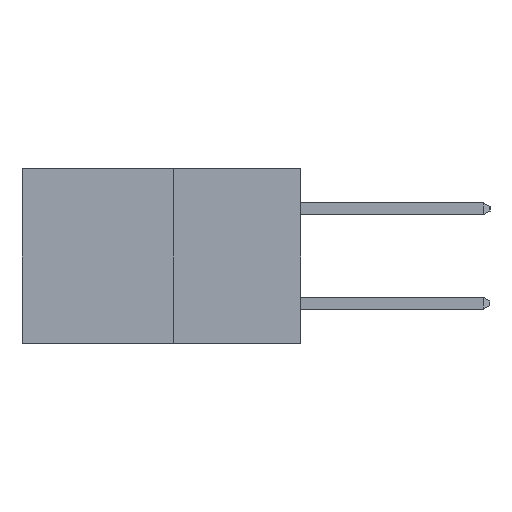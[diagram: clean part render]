
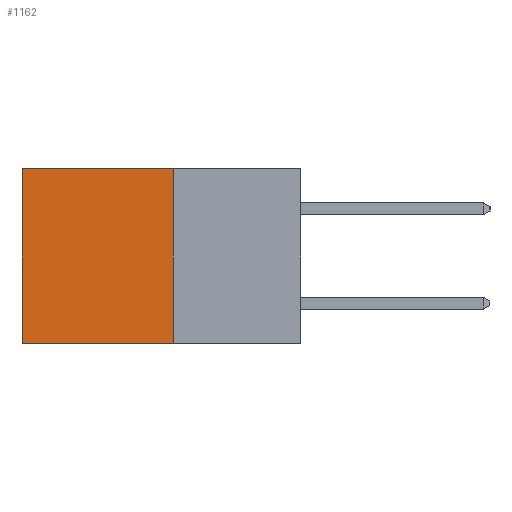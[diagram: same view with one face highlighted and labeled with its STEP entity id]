
A CAD part, left-side view. The second image highlights one B-rep face of the part: STEP entity #1162.
In plain terms, the highlighted planar face has unit normal (-1, 0, 0).
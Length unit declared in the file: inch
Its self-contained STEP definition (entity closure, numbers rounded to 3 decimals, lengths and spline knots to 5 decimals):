
#693 = VECTOR ( 'NONE', #9285, 39.37008 ) ;
#818 = VECTOR ( 'NONE', #9202, 39.37008 ) ;
#1162 = ADVANCED_FACE ( 'NONE', ( #12458 ), #6649, .F. ) ;
#2348 = EDGE_CURVE ( 'NONE', #17387, #10381, #13723, .T. ) ;
#2499 = VERTEX_POINT ( 'NONE', #16746 ) ;
#3317 = CARTESIAN_POINT ( 'NONE',  ( 0.277, 0.27, -0.37 ) ) ;
#4717 = DIRECTION ( 'NONE',  ( 1., 0., 0. ) ) ;
#5676 = LINE ( 'NONE', #15869, #693 ) ;
#5798 = LINE ( 'NONE', #7568, #818 ) ;
#5906 = CARTESIAN_POINT ( 'NONE',  ( 0.277, 0.59, 0. ) ) ;
#6201 = VECTOR ( 'NONE', #9805, 39.37008 ) ;
#6649 = PLANE ( 'NONE',  #16352 ) ;
#7479 = EDGE_CURVE ( 'NONE', #10381, #2499, #5798, .T. ) ;
#7568 = CARTESIAN_POINT ( 'NONE',  ( 0.277, 0.59, -0.37 ) ) ;
#8082 = VERTEX_POINT ( 'NONE', #10410 ) ;
#8567 = DIRECTION ( 'NONE',  ( 0., 0., -1. ) ) ;
#9202 = DIRECTION ( 'NONE',  ( 0., 0., -1. ) ) ;
#9285 = DIRECTION ( 'NONE',  ( 0., 0., -1. ) ) ;
#9293 = VECTOR ( 'NONE', #9487, 39.37008 ) ;
#9487 = DIRECTION ( 'NONE',  ( 0., 1., 0. ) ) ;
#9805 = DIRECTION ( 'NONE',  ( 0., 1., 0. ) ) ;
#9932 = CARTESIAN_POINT ( 'NONE',  ( 0.277, 0.27, 0. ) ) ;
#10321 = CARTESIAN_POINT ( 'NONE',  ( 0.277, 0.27, -0.37 ) ) ;
#10381 = VERTEX_POINT ( 'NONE', #5906 ) ;
#10410 = CARTESIAN_POINT ( 'NONE',  ( 0.277, 0.27, -0.37 ) ) ;
#10855 = EDGE_LOOP ( 'NONE', ( #17036, #16963, #16928, #16572 ) ) ;
#12458 = FACE_OUTER_BOUND ( 'NONE', #10855, .T. ) ;
#13723 = LINE ( 'NONE', #14022, #9293 ) ;
#14022 = CARTESIAN_POINT ( 'NONE',  ( 0.277, 0.27, 0. ) ) ;
#15869 = CARTESIAN_POINT ( 'NONE',  ( 0.277, 0.27, -0.37 ) ) ;
#16352 = AXIS2_PLACEMENT_3D ( 'NONE', #10321, #4717, #8567 ) ;
#16572 = ORIENTED_EDGE ( 'NONE', *, *, #2348, .T. ) ;
#16636 = EDGE_CURVE ( 'NONE', #8082, #2499, #19285, .T. ) ;
#16746 = CARTESIAN_POINT ( 'NONE',  ( 0.277, 0.59, -0.37 ) ) ;
#16928 = ORIENTED_EDGE ( 'NONE', *, *, #17122, .F. ) ;
#16963 = ORIENTED_EDGE ( 'NONE', *, *, #16636, .F. ) ;
#17036 = ORIENTED_EDGE ( 'NONE', *, *, #7479, .T. ) ;
#17122 = EDGE_CURVE ( 'NONE', #17387, #8082, #5676, .T. ) ;
#17387 = VERTEX_POINT ( 'NONE', #9932 ) ;
#19285 = LINE ( 'NONE', #3317, #6201 ) ;
